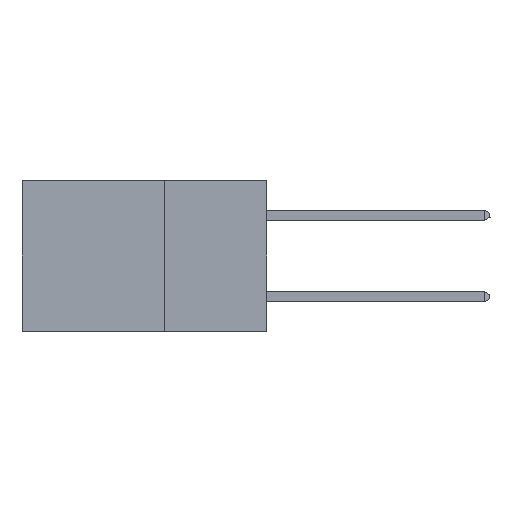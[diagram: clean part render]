
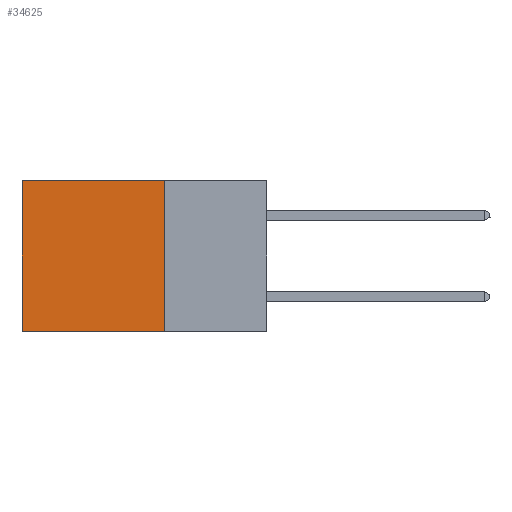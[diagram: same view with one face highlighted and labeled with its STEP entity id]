
A CAD part, left-side view. The second image highlights one B-rep face of the part: STEP entity #34625.
In plain terms, the highlighted planar face has unit normal (-1, 0, 0).
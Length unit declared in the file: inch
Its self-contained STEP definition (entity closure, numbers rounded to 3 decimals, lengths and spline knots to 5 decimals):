
#607 = DIRECTION ( 'NONE',  ( 0., 0., -1. ) ) ;
#845 = VERTEX_POINT ( 'NONE', #10544 ) ;
#1047 = CARTESIAN_POINT ( 'NONE',  ( 0.2875, 0.25, 0. ) ) ;
#2760 = VECTOR ( 'NONE', #8339, 39.37008 ) ;
#5420 = VERTEX_POINT ( 'NONE', #36951 ) ;
#6654 = EDGE_CURVE ( 'NONE', #845, #33582, #8726, .T. ) ;
#6980 = CARTESIAN_POINT ( 'NONE',  ( 0.2875, 0.25, -0.37 ) ) ;
#7094 = DIRECTION ( 'NONE',  ( 1., 0., 0. ) ) ;
#7278 = CARTESIAN_POINT ( 'NONE',  ( 0.2875, 0.25, 0. ) ) ;
#8339 = DIRECTION ( 'NONE',  ( 0., 0., -1. ) ) ;
#8726 = LINE ( 'NONE', #23555, #2760 ) ;
#8736 = CARTESIAN_POINT ( 'NONE',  ( 0.2875, 0.25, 0. ) ) ;
#10525 = VECTOR ( 'NONE', #15169, 39.37008 ) ;
#10544 = CARTESIAN_POINT ( 'NONE',  ( 0.2875, 0.6, 0. ) ) ;
#12400 = EDGE_CURVE ( 'NONE', #38035, #5420, #19057, .T. ) ;
#13113 = EDGE_LOOP ( 'NONE', ( #14518, #31774, #20560, #37891 ) ) ;
#13520 = EDGE_CURVE ( 'NONE', #38035, #845, #24709, .T. ) ;
#14518 = ORIENTED_EDGE ( 'NONE', *, *, #6654, .T. ) ;
#15169 = DIRECTION ( 'NONE',  ( 0., 1., 0. ) ) ;
#15430 = VECTOR ( 'NONE', #16508, 39.37008 ) ;
#15456 = AXIS2_PLACEMENT_3D ( 'NONE', #7278, #7094, #607 ) ;
#16508 = DIRECTION ( 'NONE',  ( 0., 0., -1. ) ) ;
#18625 = FACE_OUTER_BOUND ( 'NONE', #13113, .T. ) ;
#19057 = LINE ( 'NONE', #37028, #15430 ) ;
#19848 = VECTOR ( 'NONE', #27274, 39.37008 ) ;
#20528 = EDGE_CURVE ( 'NONE', #5420, #33582, #37059, .T. ) ;
#20560 = ORIENTED_EDGE ( 'NONE', *, *, #12400, .F. ) ;
#23555 = CARTESIAN_POINT ( 'NONE',  ( 0.2875, 0.6, 0. ) ) ;
#24709 = LINE ( 'NONE', #1047, #10525 ) ;
#27274 = DIRECTION ( 'NONE',  ( 0., 1., 0. ) ) ;
#30517 = PLANE ( 'NONE',  #15456 ) ;
#31774 = ORIENTED_EDGE ( 'NONE', *, *, #20528, .F. ) ;
#33582 = VERTEX_POINT ( 'NONE', #35580 ) ;
#34625 = ADVANCED_FACE ( 'NONE', ( #18625 ), #30517, .F. ) ;
#35580 = CARTESIAN_POINT ( 'NONE',  ( 0.2875, 0.6, -0.37 ) ) ;
#36951 = CARTESIAN_POINT ( 'NONE',  ( 0.2875, 0.25, -0.37 ) ) ;
#37028 = CARTESIAN_POINT ( 'NONE',  ( 0.2875, 0.25, 0. ) ) ;
#37059 = LINE ( 'NONE', #6980, #19848 ) ;
#37891 = ORIENTED_EDGE ( 'NONE', *, *, #13520, .T. ) ;
#38035 = VERTEX_POINT ( 'NONE', #8736 ) ;
